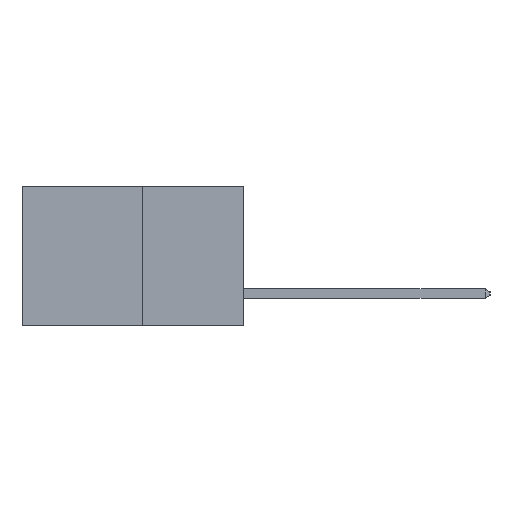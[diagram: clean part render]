
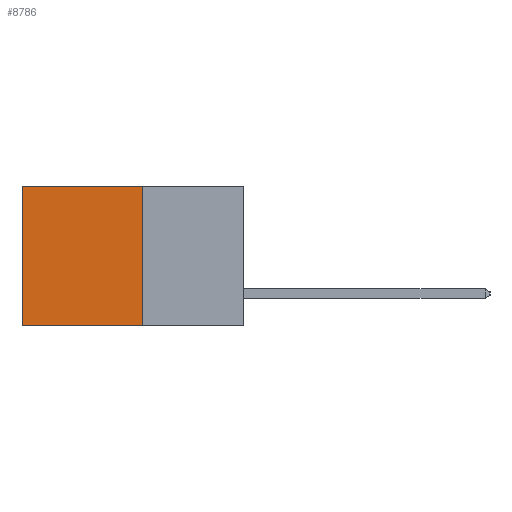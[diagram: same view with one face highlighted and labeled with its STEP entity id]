
A CAD part, left-side view. The second image highlights one B-rep face of the part: STEP entity #8786.
In plain terms, the highlighted planar face has unit normal (-1, 0, 0).
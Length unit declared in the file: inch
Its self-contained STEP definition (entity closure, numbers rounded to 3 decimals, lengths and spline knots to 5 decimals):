
#954 = DIRECTION ( 'NONE',  ( 0., 0., -1. ) ) ;
#1474 = VERTEX_POINT ( 'NONE', #5082 ) ;
#1760 = CARTESIAN_POINT ( 'NONE',  ( 0.277, 0.59, 0. ) ) ;
#1774 = CARTESIAN_POINT ( 'NONE',  ( 0.277, 0.59, -0.37 ) ) ;
#1969 = EDGE_CURVE ( 'NONE', #1474, #7714, #6312, .T. ) ;
#2223 = ORIENTED_EDGE ( 'NONE', *, *, #5653, .F. ) ;
#2359 = ORIENTED_EDGE ( 'NONE', *, *, #3841, .T. ) ;
#2438 = VECTOR ( 'NONE', #6390, 39.37008 ) ;
#2760 = LINE ( 'NONE', #6696, #6384 ) ;
#3058 = CARTESIAN_POINT ( 'NONE',  ( 0.277, 0.27, -0.37 ) ) ;
#3314 = AXIS2_PLACEMENT_3D ( 'NONE', #5927, #5634, #5684 ) ;
#3841 = EDGE_CURVE ( 'NONE', #7714, #5666, #6280, .T. ) ;
#4195 = CARTESIAN_POINT ( 'NONE',  ( 0.277, 0.27, -0.37 ) ) ;
#4240 = LINE ( 'NONE', #4195, #7761 ) ;
#5082 = CARTESIAN_POINT ( 'NONE',  ( 0.277, 0.27, 0. ) ) ;
#5634 = DIRECTION ( 'NONE',  ( 1., 0., 0. ) ) ;
#5653 = EDGE_CURVE ( 'NONE', #8089, #5666, #4240, .T. ) ;
#5666 = VERTEX_POINT ( 'NONE', #1774 ) ;
#5684 = DIRECTION ( 'NONE',  ( 0., 0., -1. ) ) ;
#5724 = PLANE ( 'NONE',  #3314 ) ;
#5927 = CARTESIAN_POINT ( 'NONE',  ( 0.277, 0.27, -0.37 ) ) ;
#6169 = FACE_OUTER_BOUND ( 'NONE', #6498, .T. ) ;
#6280 = LINE ( 'NONE', #9111, #8101 ) ;
#6312 = LINE ( 'NONE', #7516, #2438 ) ;
#6384 = VECTOR ( 'NONE', #6589, 39.37008 ) ;
#6390 = DIRECTION ( 'NONE',  ( 0., 1., 0. ) ) ;
#6498 = EDGE_LOOP ( 'NONE', ( #2359, #2223, #8875, #7607 ) ) ;
#6589 = DIRECTION ( 'NONE',  ( 0., 0., -1. ) ) ;
#6696 = CARTESIAN_POINT ( 'NONE',  ( 0.277, 0.27, -0.37 ) ) ;
#7516 = CARTESIAN_POINT ( 'NONE',  ( 0.277, 0.27, 0. ) ) ;
#7607 = ORIENTED_EDGE ( 'NONE', *, *, #1969, .T. ) ;
#7714 = VERTEX_POINT ( 'NONE', #1760 ) ;
#7761 = VECTOR ( 'NONE', #8352, 39.37008 ) ;
#8089 = VERTEX_POINT ( 'NONE', #3058 ) ;
#8101 = VECTOR ( 'NONE', #954, 39.37008 ) ;
#8352 = DIRECTION ( 'NONE',  ( 0., 1., 0. ) ) ;
#8744 = EDGE_CURVE ( 'NONE', #1474, #8089, #2760, .T. ) ;
#8786 = ADVANCED_FACE ( 'NONE', ( #6169 ), #5724, .F. ) ;
#8875 = ORIENTED_EDGE ( 'NONE', *, *, #8744, .F. ) ;
#9111 = CARTESIAN_POINT ( 'NONE',  ( 0.277, 0.59, -0.37 ) ) ;
